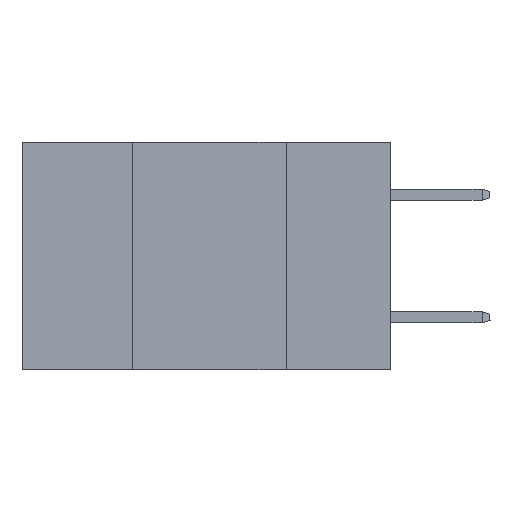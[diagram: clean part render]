
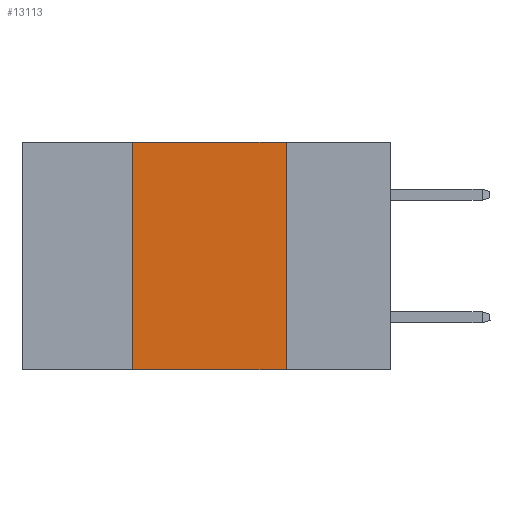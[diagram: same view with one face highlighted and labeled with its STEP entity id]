
A CAD part, left-side view. The second image highlights one B-rep face of the part: STEP entity #13113.
In plain terms, the highlighted planar face has unit normal (-1, 0, 0).
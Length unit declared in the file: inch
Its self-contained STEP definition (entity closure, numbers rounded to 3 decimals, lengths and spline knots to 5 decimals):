
#160 = CARTESIAN_POINT ( 'NONE',  ( 0., 0.42, -0.37 ) ) ;
#700 = CARTESIAN_POINT ( 'NONE',  ( 0., 0.42, 0. ) ) ;
#1113 = LINE ( 'NONE', #9033, #10891 ) ;
#1334 = ORIENTED_EDGE ( 'NONE', *, *, #17947, .T. ) ;
#1912 = CARTESIAN_POINT ( 'NONE',  ( 0., 0.42, 0. ) ) ;
#2570 = DIRECTION ( 'NONE',  ( 0., 0., 1. ) ) ;
#2775 = CARTESIAN_POINT ( 'NONE',  ( 0., 0.6, 0. ) ) ;
#4558 = PLANE ( 'NONE',  #6388 ) ;
#5498 = LINE ( 'NONE', #16334, #8609 ) ;
#5550 = ORIENTED_EDGE ( 'NONE', *, *, #6507, .F. ) ;
#5676 = VERTEX_POINT ( 'NONE', #160 ) ;
#6388 = AXIS2_PLACEMENT_3D ( 'NONE', #8158, #20687, #10080 ) ;
#6507 = EDGE_CURVE ( 'NONE', #5676, #19632, #11611, .T. ) ;
#8158 = CARTESIAN_POINT ( 'NONE',  ( 0., 0.6, 0. ) ) ;
#8609 = VECTOR ( 'NONE', #18082, 39.37008 ) ;
#8955 = EDGE_CURVE ( 'NONE', #9113, #18453, #5498, .T. ) ;
#9033 = CARTESIAN_POINT ( 'NONE',  ( 0., 0.6, -0.37 ) ) ;
#9113 = VERTEX_POINT ( 'NONE', #11353 ) ;
#9995 = EDGE_LOOP ( 'NONE', ( #17102, #21198, #5550, #1334 ) ) ;
#10080 = DIRECTION ( 'NONE',  ( 0., 0., -1. ) ) ;
#10572 = CARTESIAN_POINT ( 'NONE',  ( 0., 0.17, -0.37 ) ) ;
#10891 = VECTOR ( 'NONE', #21451, 39.37008 ) ;
#11353 = CARTESIAN_POINT ( 'NONE',  ( 0., 0.17, 0. ) ) ;
#11611 = LINE ( 'NONE', #700, #15802 ) ;
#13113 = ADVANCED_FACE ( 'NONE', ( #14068 ), #4558, .F. ) ;
#13156 = EDGE_CURVE ( 'NONE', #19632, #9113, #13536, .T. ) ;
#13536 = LINE ( 'NONE', #2775, #19316 ) ;
#14068 = FACE_OUTER_BOUND ( 'NONE', #9995, .T. ) ;
#15802 = VECTOR ( 'NONE', #2570, 39.37008 ) ;
#16334 = CARTESIAN_POINT ( 'NONE',  ( 0., 0.17, 0. ) ) ;
#17102 = ORIENTED_EDGE ( 'NONE', *, *, #8955, .F. ) ;
#17315 = DIRECTION ( 'NONE',  ( 0., -1., 0. ) ) ;
#17947 = EDGE_CURVE ( 'NONE', #5676, #18453, #1113, .T. ) ;
#18082 = DIRECTION ( 'NONE',  ( 0., 0., -1. ) ) ;
#18453 = VERTEX_POINT ( 'NONE', #10572 ) ;
#19316 = VECTOR ( 'NONE', #17315, 39.37008 ) ;
#19632 = VERTEX_POINT ( 'NONE', #1912 ) ;
#20687 = DIRECTION ( 'NONE',  ( 1., 0., 0. ) ) ;
#21198 = ORIENTED_EDGE ( 'NONE', *, *, #13156, .F. ) ;
#21451 = DIRECTION ( 'NONE',  ( 0., -1., 0. ) ) ;
